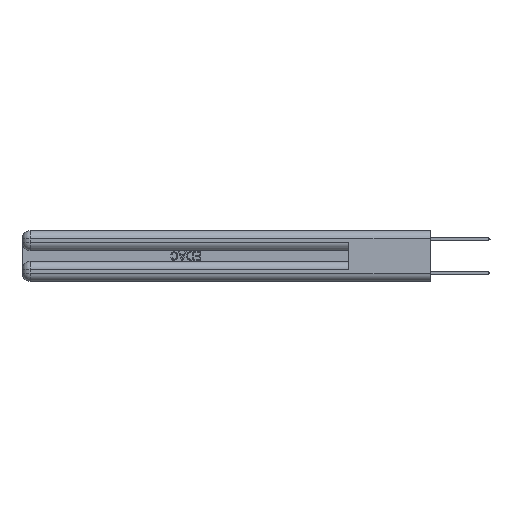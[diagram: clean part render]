
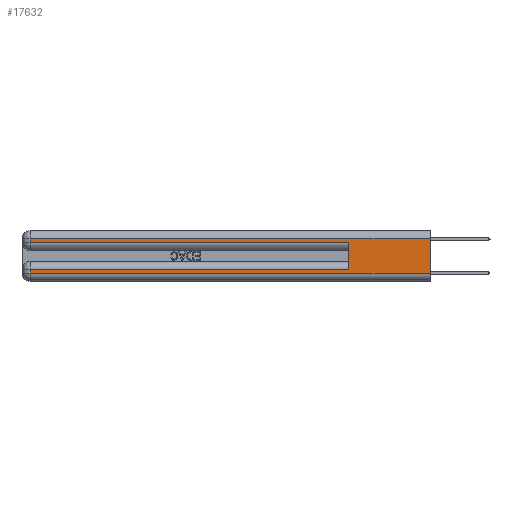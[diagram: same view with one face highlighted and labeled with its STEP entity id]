
A CAD part, left-side view. The second image highlights one B-rep face of the part: STEP entity #17632.
In plain terms, the highlighted planar face has unit normal (-1, 0, 0).
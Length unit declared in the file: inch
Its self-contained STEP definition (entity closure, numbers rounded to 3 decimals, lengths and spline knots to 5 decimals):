
#264 = CARTESIAN_POINT ( 'NONE',  ( 0., 0., 0.06 ) ) ;
#830 = EDGE_LOOP ( 'NONE', ( #4177, #6667, #7955, #11927, #17038, #3208, #16213, #26318 ) ) ;
#846 = CARTESIAN_POINT ( 'NONE',  ( 0., 0., 0.285 ) ) ;
#1010 = CARTESIAN_POINT ( 'NONE',  ( 0., 2.94, 0.085 ) ) ;
#1966 = EDGE_CURVE ( 'NONE', #6137, #21453, #16723, .T. ) ;
#2276 = EDGE_CURVE ( 'NONE', #6137, #5340, #3740, .T. ) ;
#2678 = CARTESIAN_POINT ( 'NONE',  ( 0., 2.94, 0.285 ) ) ;
#2850 = CARTESIAN_POINT ( 'NONE',  ( 0., 0.6, 0.085 ) ) ;
#3208 = ORIENTED_EDGE ( 'NONE', *, *, #3816, .T. ) ;
#3440 = CARTESIAN_POINT ( 'NONE',  ( 0., 0., 0.31 ) ) ;
#3740 = LINE ( 'NONE', #11269, #15616 ) ;
#3816 = EDGE_CURVE ( 'NONE', #27109, #26619, #17188, .T. ) ;
#3825 = LINE ( 'NONE', #20804, #7299 ) ;
#4177 = ORIENTED_EDGE ( 'NONE', *, *, #1966, .F. ) ;
#4384 = LINE ( 'NONE', #17566, #26806 ) ;
#5204 = CARTESIAN_POINT ( 'NONE',  ( 0., 0., 0.37 ) ) ;
#5340 = VERTEX_POINT ( 'NONE', #24901 ) ;
#6004 = DIRECTION ( 'NONE',  ( 0., 0., -1. ) ) ;
#6125 = CARTESIAN_POINT ( 'NONE',  ( 0., 0., 0.37 ) ) ;
#6137 = VERTEX_POINT ( 'NONE', #3440 ) ;
#6297 = VERTEX_POINT ( 'NONE', #25182 ) ;
#6667 = ORIENTED_EDGE ( 'NONE', *, *, #2276, .T. ) ;
#6951 = VECTOR ( 'NONE', #11153, 39.37008 ) ;
#7299 = VECTOR ( 'NONE', #21098, 39.37008 ) ;
#7955 = ORIENTED_EDGE ( 'NONE', *, *, #20928, .T. ) ;
#9456 = VECTOR ( 'NONE', #9837, 39.37008 ) ;
#9837 = DIRECTION ( 'NONE',  ( 0., 1., 0. ) ) ;
#10419 = VECTOR ( 'NONE', #15219, 39.37008 ) ;
#10934 = VERTEX_POINT ( 'NONE', #14850 ) ;
#11153 = DIRECTION ( 'NONE',  ( 0., -1., 0. ) ) ;
#11269 = CARTESIAN_POINT ( 'NONE',  ( 0., 0., 0.31 ) ) ;
#11773 = CARTESIAN_POINT ( 'NONE',  ( 0., 0., 0.085 ) ) ;
#11927 = ORIENTED_EDGE ( 'NONE', *, *, #27766, .T. ) ;
#12007 = DIRECTION ( 'NONE',  ( 0., -1., 0. ) ) ;
#12375 = DIRECTION ( 'NONE',  ( 1., 0., 0. ) ) ;
#13526 = AXIS2_PLACEMENT_3D ( 'NONE', #5204, #12375, #21380 ) ;
#13858 = CARTESIAN_POINT ( 'NONE',  ( 0., 2.94, 0.37 ) ) ;
#14169 = PLANE ( 'NONE',  #13526 ) ;
#14850 = CARTESIAN_POINT ( 'NONE',  ( 0., 2.94, 0.06 ) ) ;
#14961 = VECTOR ( 'NONE', #12007, 39.37008 ) ;
#14983 = EDGE_CURVE ( 'NONE', #10934, #21453, #20276, .T. ) ;
#15219 = DIRECTION ( 'NONE',  ( 0., 0., -1. ) ) ;
#15616 = VECTOR ( 'NONE', #16150, 39.37008 ) ;
#16150 = DIRECTION ( 'NONE',  ( 0., 1., 0. ) ) ;
#16205 = DIRECTION ( 'NONE',  ( 0., 0., -1. ) ) ;
#16213 = ORIENTED_EDGE ( 'NONE', *, *, #27846, .T. ) ;
#16699 = VECTOR ( 'NONE', #16205, 39.37008 ) ;
#16723 = LINE ( 'NONE', #6125, #10419 ) ;
#17038 = ORIENTED_EDGE ( 'NONE', *, *, #26469, .F. ) ;
#17188 = LINE ( 'NONE', #11773, #9456 ) ;
#17566 = CARTESIAN_POINT ( 'NONE',  ( 0., 2.94, 0.37 ) ) ;
#17632 = ADVANCED_FACE ( 'NONE', ( #19584 ), #14169, .F. ) ;
#18827 = CARTESIAN_POINT ( 'NONE',  ( 0., 0., 0.06 ) ) ;
#19584 = FACE_OUTER_BOUND ( 'NONE', #830, .T. ) ;
#20276 = LINE ( 'NONE', #18827, #6951 ) ;
#20804 = CARTESIAN_POINT ( 'NONE',  ( 0., 0.6, 0.145 ) ) ;
#20928 = EDGE_CURVE ( 'NONE', #5340, #22256, #4384, .T. ) ;
#21098 = DIRECTION ( 'NONE',  ( 0., 0., 1. ) ) ;
#21380 = DIRECTION ( 'NONE',  ( 0., 0., -1. ) ) ;
#21453 = VERTEX_POINT ( 'NONE', #264 ) ;
#22256 = VERTEX_POINT ( 'NONE', #2678 ) ;
#24901 = CARTESIAN_POINT ( 'NONE',  ( 0., 2.94, 0.31 ) ) ;
#25182 = CARTESIAN_POINT ( 'NONE',  ( 0., 0.6, 0.285 ) ) ;
#26176 = LINE ( 'NONE', #846, #14961 ) ;
#26318 = ORIENTED_EDGE ( 'NONE', *, *, #14983, .T. ) ;
#26469 = EDGE_CURVE ( 'NONE', #27109, #6297, #3825, .T. ) ;
#26619 = VERTEX_POINT ( 'NONE', #1010 ) ;
#26806 = VECTOR ( 'NONE', #6004, 39.37008 ) ;
#27109 = VERTEX_POINT ( 'NONE', #2850 ) ;
#27611 = LINE ( 'NONE', #13858, #16699 ) ;
#27766 = EDGE_CURVE ( 'NONE', #22256, #6297, #26176, .T. ) ;
#27846 = EDGE_CURVE ( 'NONE', #26619, #10934, #27611, .T. ) ;
